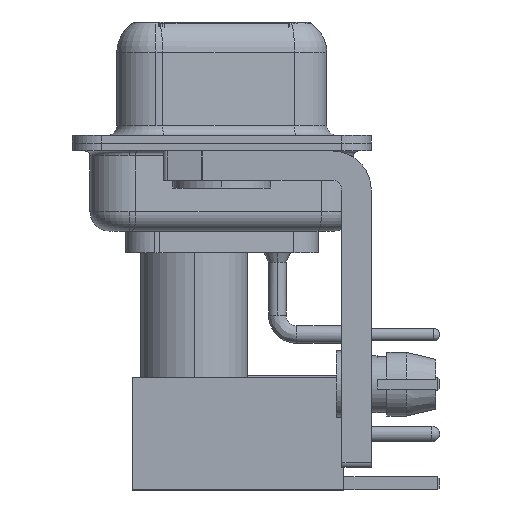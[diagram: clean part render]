
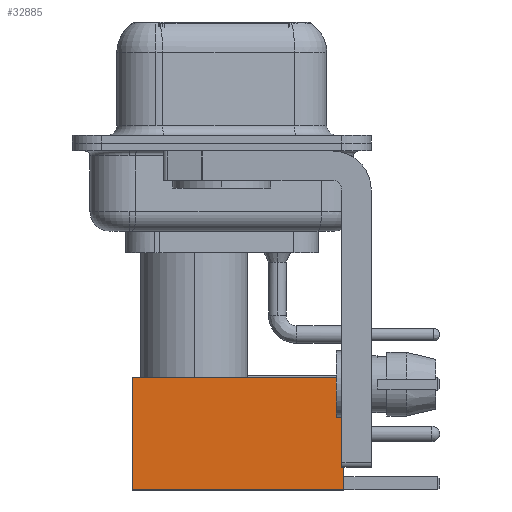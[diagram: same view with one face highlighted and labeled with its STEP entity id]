
A CAD part, left-side view. The second image highlights one B-rep face of the part: STEP entity #32885.
In plain terms, the highlighted face is planar.
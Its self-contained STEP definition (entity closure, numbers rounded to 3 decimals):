
#2295 = VECTOR ( 'NONE', #18753, 1000. ) ;
#2389 = VECTOR ( 'NONE', #22948, 1000. ) ;
#5756 = EDGE_CURVE ( 'NONE', #8787, #31700, #29945, .T. ) ;
#6755 = ORIENTED_EDGE ( 'NONE', *, *, #5756, .T. ) ;
#7128 = CARTESIAN_POINT ( 'NONE',  ( 2.875, 2.875, 0. ) ) ;
#7182 = DIRECTION ( 'NONE',  ( 0., 0., -1. ) ) ;
#7915 = CARTESIAN_POINT ( 'NONE',  ( 2.875, 2.875, 0. ) ) ;
#7985 = LINE ( 'NONE', #12861, #11322 ) ;
#8787 = VERTEX_POINT ( 'NONE', #11056 ) ;
#11056 = CARTESIAN_POINT ( 'NONE',  ( 2.875, 2.875, 10.82 ) ) ;
#11322 = VECTOR ( 'NONE', #27112, 1000. ) ;
#11863 = CARTESIAN_POINT ( 'NONE',  ( -2.875, 2.875, 0. ) ) ;
#12107 = EDGE_CURVE ( 'NONE', #23655, #16057, #17674, .T. ) ;
#12861 = CARTESIAN_POINT ( 'NONE',  ( 0., 2.875, 10.82 ) ) ;
#12879 = ORIENTED_EDGE ( 'NONE', *, *, #23622, .T. ) ;
#14549 = DIRECTION ( 'NONE',  ( 0., 1., 0. ) ) ;
#15136 = CARTESIAN_POINT ( 'NONE',  ( -2.875, 2.875, 0. ) ) ;
#15432 = CARTESIAN_POINT ( 'NONE',  ( 2.875, 2.875, 0. ) ) ;
#16057 = VERTEX_POINT ( 'NONE', #11863 ) ;
#17674 = LINE ( 'NONE', #15136, #35419 ) ;
#18753 = DIRECTION ( 'NONE',  ( 0., 0., -1. ) ) ;
#22236 = CARTESIAN_POINT ( 'NONE',  ( -2.875, 2.875, 10.82 ) ) ;
#22948 = DIRECTION ( 'NONE',  ( -1., 0., 0. ) ) ;
#23622 = EDGE_CURVE ( 'NONE', #31700, #16057, #25487, .T. ) ;
#23655 = VERTEX_POINT ( 'NONE', #22236 ) ;
#25487 = LINE ( 'NONE', #31072, #2389 ) ;
#25561 = DIRECTION ( 'NONE',  ( 0., 0., 1. ) ) ;
#27112 = DIRECTION ( 'NONE',  ( -1., 0., 0. ) ) ;
#28823 = EDGE_CURVE ( 'NONE', #8787, #23655, #7985, .T. ) ;
#29168 = FACE_OUTER_BOUND ( 'NONE', #35081, .T. ) ;
#29945 = LINE ( 'NONE', #7915, #2295 ) ;
#30492 = AXIS2_PLACEMENT_3D ( 'NONE', #7128, #14549, #25561 ) ;
#31072 = CARTESIAN_POINT ( 'NONE',  ( 0., 2.875, 0. ) ) ;
#31549 = ORIENTED_EDGE ( 'NONE', *, *, #28823, .F. ) ;
#31700 = VERTEX_POINT ( 'NONE', #15432 ) ;
#31866 = PLANE ( 'NONE',  #30492 ) ;
#32016 = ORIENTED_EDGE ( 'NONE', *, *, #12107, .F. ) ;
#32885 = ADVANCED_FACE ( 'NONE', ( #29168 ), #31866, .T. ) ;
#35081 = EDGE_LOOP ( 'NONE', ( #6755, #12879, #32016, #31549 ) ) ;
#35419 = VECTOR ( 'NONE', #7182, 1000. ) ;
